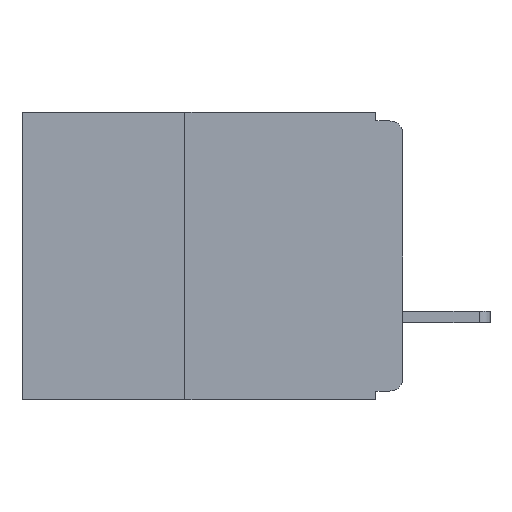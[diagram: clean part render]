
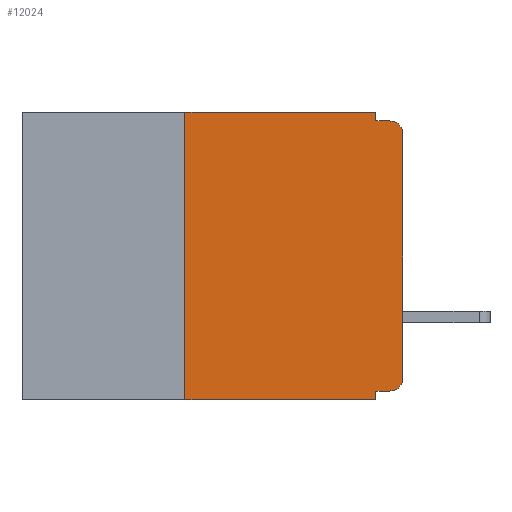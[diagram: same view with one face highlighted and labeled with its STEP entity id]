
A CAD part, left-side view. The second image highlights one B-rep face of the part: STEP entity #12024.
In plain terms, the highlighted planar face has unit normal (-1, 0, 0).
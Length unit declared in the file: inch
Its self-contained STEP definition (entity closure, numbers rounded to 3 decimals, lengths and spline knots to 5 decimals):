
#37 = AXIS2_PLACEMENT_3D ( 'NONE', #6912, #17126, #8388 ) ;
#203 = DIRECTION ( 'NONE',  ( 0., 0., -1. ) ) ;
#364 = LINE ( 'NONE', #3446, #7967 ) ;
#449 = CARTESIAN_POINT ( 'NONE',  ( 0., 0., -0.025 ) ) ;
#477 = AXIS2_PLACEMENT_3D ( 'NONE', #7792, #9256, #203 ) ;
#936 = VERTEX_POINT ( 'NONE', #3798 ) ;
#1219 = VERTEX_POINT ( 'NONE', #10732 ) ;
#1365 = CARTESIAN_POINT ( 'NONE',  ( 0., 0., 0. ) ) ;
#1471 = VERTEX_POINT ( 'NONE', #2036 ) ;
#1618 = DIRECTION ( 'NONE',  ( 0., 0., -1. ) ) ;
#1951 = CARTESIAN_POINT ( 'NONE',  ( 0., 0.25, -0.33 ) ) ;
#1998 = VERTEX_POINT ( 'NONE', #14596 ) ;
#2036 = CARTESIAN_POINT ( 'NONE',  ( 0., 0.031, -0.32 ) ) ;
#2063 = FACE_OUTER_BOUND ( 'NONE', #6497, .T. ) ;
#2086 = LINE ( 'NONE', #11857, #9604 ) ;
#2139 = ORIENTED_EDGE ( 'NONE', *, *, #16441, .T. ) ;
#2538 = LINE ( 'NONE', #6089, #10008 ) ;
#2648 = ORIENTED_EDGE ( 'NONE', *, *, #8014, .T. ) ;
#2675 = VECTOR ( 'NONE', #16762, 39.37008 ) ;
#2932 = DIRECTION ( 'NONE',  ( 0., 0., 1. ) ) ;
#2980 = EDGE_CURVE ( 'NONE', #1998, #18289, #8996, .T. ) ;
#3446 = CARTESIAN_POINT ( 'NONE',  ( 0., 0., -0.32 ) ) ;
#3798 = CARTESIAN_POINT ( 'NONE',  ( 0., 0.031, 0. ) ) ;
#4237 = CARTESIAN_POINT ( 'NONE',  ( 0., 0.031, -0.01 ) ) ;
#4856 = DIRECTION ( 'NONE',  ( 0., 0., -1. ) ) ;
#4922 = CARTESIAN_POINT ( 'NONE',  ( 0., 0.031, -0.33 ) ) ;
#5245 = CARTESIAN_POINT ( 'NONE',  ( 0., 0.015, -0.305 ) ) ;
#5628 = EDGE_CURVE ( 'NONE', #5921, #13639, #2086, .T. ) ;
#5690 = DIRECTION ( 'NONE',  ( 0., -1., 0. ) ) ;
#5694 = DIRECTION ( 'NONE',  ( -1., 0., 0. ) ) ;
#5866 = EDGE_CURVE ( 'NONE', #1471, #12121, #17599, .T. ) ;
#5921 = VERTEX_POINT ( 'NONE', #4237 ) ;
#6089 = CARTESIAN_POINT ( 'NONE',  ( 0., 0.437, 0. ) ) ;
#6497 = EDGE_LOOP ( 'NONE', ( #2139, #2648, #10575, #7143, #14877, #18740, #19171, #8058, #15824, #8512 ) ) ;
#6565 = CARTESIAN_POINT ( 'NONE',  ( 0., 0.031, -0.33 ) ) ;
#6888 = EDGE_CURVE ( 'NONE', #15783, #12121, #16619, .T. ) ;
#6912 = CARTESIAN_POINT ( 'NONE',  ( 0., 0.015, -0.025 ) ) ;
#7031 = EDGE_CURVE ( 'NONE', #1219, #936, #2538, .T. ) ;
#7143 = ORIENTED_EDGE ( 'NONE', *, *, #10824, .F. ) ;
#7219 = CARTESIAN_POINT ( 'NONE',  ( 0., 0.437, -0.33 ) ) ;
#7792 = CARTESIAN_POINT ( 'NONE',  ( 0., 0.437, 0. ) ) ;
#7818 = LINE ( 'NONE', #17704, #18945 ) ;
#7952 = CARTESIAN_POINT ( 'NONE',  ( 0., 0., -0.305 ) ) ;
#7967 = VECTOR ( 'NONE', #18114, 39.37008 ) ;
#8014 = EDGE_CURVE ( 'NONE', #15542, #13639, #11790, .T. ) ;
#8058 = ORIENTED_EDGE ( 'NONE', *, *, #5866, .F. ) ;
#8388 = DIRECTION ( 'NONE',  ( 0., 0., -1. ) ) ;
#8512 = ORIENTED_EDGE ( 'NONE', *, *, #2980, .T. ) ;
#8996 = CIRCLE ( 'NONE', #15807, 0.015 ) ;
#9256 = DIRECTION ( 'NONE',  ( 1., 0., 0. ) ) ;
#9604 = VECTOR ( 'NONE', #10977, 39.37008 ) ;
#9830 = VECTOR ( 'NONE', #4856, 39.37008 ) ;
#9838 = EDGE_CURVE ( 'NONE', #15783, #1219, #18327, .T. ) ;
#10008 = VECTOR ( 'NONE', #13352, 39.37008 ) ;
#10461 = VECTOR ( 'NONE', #2932, 39.37008 ) ;
#10575 = ORIENTED_EDGE ( 'NONE', *, *, #5628, .F. ) ;
#10732 = CARTESIAN_POINT ( 'NONE',  ( 0., 0.25, 0. ) ) ;
#10824 = EDGE_CURVE ( 'NONE', #936, #5921, #7818, .T. ) ;
#10977 = DIRECTION ( 'NONE',  ( 0., -1., 0. ) ) ;
#11790 = CIRCLE ( 'NONE', #37, 0.015 ) ;
#11857 = CARTESIAN_POINT ( 'NONE',  ( 0., 0., -0.01 ) ) ;
#12024 = ADVANCED_FACE ( 'NONE', ( #2063 ), #16511, .F. ) ;
#12121 = VERTEX_POINT ( 'NONE', #6565 ) ;
#12766 = VECTOR ( 'NONE', #5690, 39.37008 ) ;
#13352 = DIRECTION ( 'NONE',  ( 0., -1., 0. ) ) ;
#13639 = VERTEX_POINT ( 'NONE', #16027 ) ;
#14596 = CARTESIAN_POINT ( 'NONE',  ( 0., 0.015, -0.32 ) ) ;
#14834 = EDGE_CURVE ( 'NONE', #1998, #1471, #364, .T. ) ;
#14877 = ORIENTED_EDGE ( 'NONE', *, *, #7031, .F. ) ;
#15542 = VERTEX_POINT ( 'NONE', #449 ) ;
#15783 = VERTEX_POINT ( 'NONE', #15987 ) ;
#15807 = AXIS2_PLACEMENT_3D ( 'NONE', #5245, #5694, #1618 ) ;
#15824 = ORIENTED_EDGE ( 'NONE', *, *, #14834, .F. ) ;
#15987 = CARTESIAN_POINT ( 'NONE',  ( 0., 0.25, -0.33 ) ) ;
#16027 = CARTESIAN_POINT ( 'NONE',  ( 0., 0.015, -0.01 ) ) ;
#16441 = EDGE_CURVE ( 'NONE', #18289, #15542, #17756, .T. ) ;
#16511 = PLANE ( 'NONE',  #477 ) ;
#16619 = LINE ( 'NONE', #7219, #12766 ) ;
#16762 = DIRECTION ( 'NONE',  ( 0., 0., 1. ) ) ;
#17126 = DIRECTION ( 'NONE',  ( -1., 0., 0. ) ) ;
#17599 = LINE ( 'NONE', #4922, #9830 ) ;
#17704 = CARTESIAN_POINT ( 'NONE',  ( 0., 0.031, 0. ) ) ;
#17756 = LINE ( 'NONE', #1365, #10461 ) ;
#18114 = DIRECTION ( 'NONE',  ( 0., 1., 0. ) ) ;
#18289 = VERTEX_POINT ( 'NONE', #7952 ) ;
#18327 = LINE ( 'NONE', #1951, #2675 ) ;
#18740 = ORIENTED_EDGE ( 'NONE', *, *, #9838, .F. ) ;
#18945 = VECTOR ( 'NONE', #19101, 39.37008 ) ;
#19101 = DIRECTION ( 'NONE',  ( 0., 0., -1. ) ) ;
#19171 = ORIENTED_EDGE ( 'NONE', *, *, #6888, .T. ) ;
